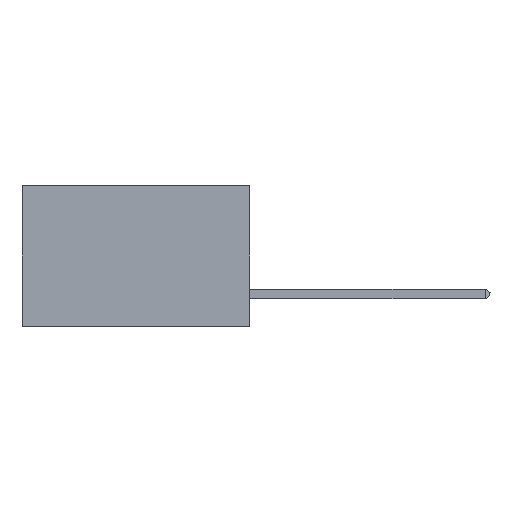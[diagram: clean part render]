
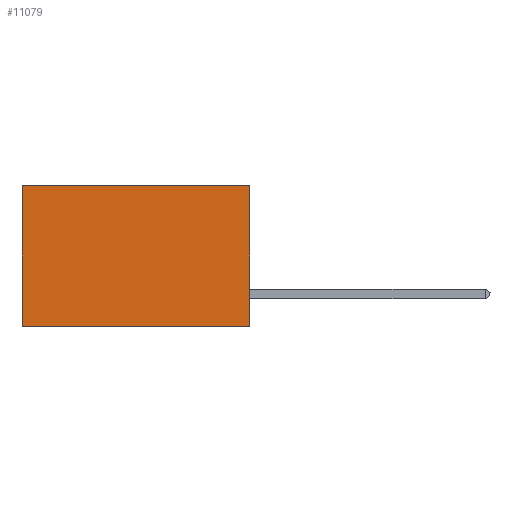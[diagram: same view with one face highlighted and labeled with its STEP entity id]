
A CAD part, left-side view. The second image highlights one B-rep face of the part: STEP entity #11079.
In plain terms, the highlighted planar face has unit normal (-1, 0, 0).
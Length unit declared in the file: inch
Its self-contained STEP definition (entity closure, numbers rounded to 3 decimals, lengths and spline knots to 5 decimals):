
#1270 = CARTESIAN_POINT ( 'NONE',  ( 0.2875, 0., 0. ) ) ;
#1654 = VECTOR ( 'NONE', #12601, 39.37008 ) ;
#1999 = CARTESIAN_POINT ( 'NONE',  ( 0.2875, 0., 0. ) ) ;
#3090 = EDGE_CURVE ( 'NONE', #18165, #20658, #22932, .T. ) ;
#4450 = PLANE ( 'NONE',  #12389 ) ;
#4573 = EDGE_CURVE ( 'NONE', #8710, #20658, #9508, .T. ) ;
#5561 = DIRECTION ( 'NONE',  ( 0., 1., 0. ) ) ;
#7636 = ORIENTED_EDGE ( 'NONE', *, *, #4573, .F. ) ;
#8415 = LINE ( 'NONE', #1270, #15246 ) ;
#8657 = CARTESIAN_POINT ( 'NONE',  ( 0.2875, 0., 0. ) ) ;
#8710 = VERTEX_POINT ( 'NONE', #12132 ) ;
#9508 = LINE ( 'NONE', #10670, #1654 ) ;
#10670 = CARTESIAN_POINT ( 'NONE',  ( 0.2875, 0., -0.37 ) ) ;
#11079 = ADVANCED_FACE ( 'NONE', ( #19406 ), #4450, .F. ) ;
#12132 = CARTESIAN_POINT ( 'NONE',  ( 0.2875, 0., -0.37 ) ) ;
#12389 = AXIS2_PLACEMENT_3D ( 'NONE', #8657, #13026, #23198 ) ;
#12601 = DIRECTION ( 'NONE',  ( 0., 1., 0. ) ) ;
#13026 = DIRECTION ( 'NONE',  ( 1., 0., 0. ) ) ;
#14757 = EDGE_CURVE ( 'NONE', #23994, #8710, #8415, .T. ) ;
#15246 = VECTOR ( 'NONE', #25989, 39.37008 ) ;
#16617 = CARTESIAN_POINT ( 'NONE',  ( 0.2875, 0., 0. ) ) ;
#17899 = LINE ( 'NONE', #16617, #26365 ) ;
#17934 = ORIENTED_EDGE ( 'NONE', *, *, #22462, .T. ) ;
#18165 = VERTEX_POINT ( 'NONE', #21392 ) ;
#18232 = ORIENTED_EDGE ( 'NONE', *, *, #14757, .F. ) ;
#19406 = FACE_OUTER_BOUND ( 'NONE', #20271, .T. ) ;
#20042 = VECTOR ( 'NONE', #21649, 39.37008 ) ;
#20271 = EDGE_LOOP ( 'NONE', ( #25396, #7636, #18232, #17934 ) ) ;
#20658 = VERTEX_POINT ( 'NONE', #25212 ) ;
#21392 = CARTESIAN_POINT ( 'NONE',  ( 0.2875, 0.6, 0. ) ) ;
#21649 = DIRECTION ( 'NONE',  ( 0., 0., -1. ) ) ;
#21909 = CARTESIAN_POINT ( 'NONE',  ( 0.2875, 0.6, 0. ) ) ;
#22462 = EDGE_CURVE ( 'NONE', #23994, #18165, #17899, .T. ) ;
#22932 = LINE ( 'NONE', #21909, #20042 ) ;
#23198 = DIRECTION ( 'NONE',  ( 0., 0., -1. ) ) ;
#23994 = VERTEX_POINT ( 'NONE', #1999 ) ;
#25212 = CARTESIAN_POINT ( 'NONE',  ( 0.2875, 0.6, -0.37 ) ) ;
#25396 = ORIENTED_EDGE ( 'NONE', *, *, #3090, .T. ) ;
#25989 = DIRECTION ( 'NONE',  ( 0., 0., -1. ) ) ;
#26365 = VECTOR ( 'NONE', #5561, 39.37008 ) ;
